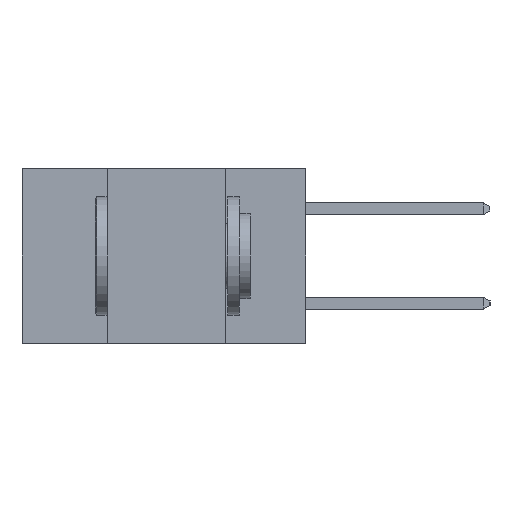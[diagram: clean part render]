
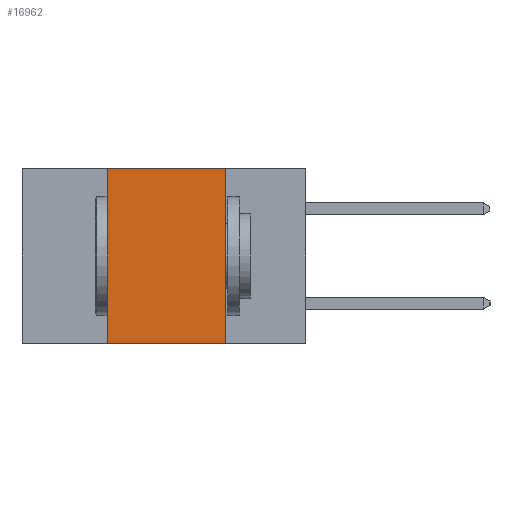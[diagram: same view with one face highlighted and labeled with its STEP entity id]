
A CAD part, left-side view. The second image highlights one B-rep face of the part: STEP entity #16962.
In plain terms, the highlighted planar face has unit normal (-1, 0, 0).
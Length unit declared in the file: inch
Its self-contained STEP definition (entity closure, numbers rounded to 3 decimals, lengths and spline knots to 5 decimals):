
#395 = CARTESIAN_POINT ( 'NONE',  ( 0., 0.17, -0.37 ) ) ;
#1537 = CARTESIAN_POINT ( 'NONE',  ( 0., 0.42, -0.37 ) ) ;
#2744 = VECTOR ( 'NONE', #6840, 39.37008 ) ;
#3295 = EDGE_CURVE ( 'NONE', #20723, #13925, #17741, .T. ) ;
#4956 = LINE ( 'NONE', #1537, #2744 ) ;
#6370 = ORIENTED_EDGE ( 'NONE', *, *, #20354, .F. ) ;
#6571 = VERTEX_POINT ( 'NONE', #9847 ) ;
#6707 = EDGE_CURVE ( 'NONE', #20723, #6571, #4956, .T. ) ;
#6840 = DIRECTION ( 'NONE',  ( 0., 0., 1. ) ) ;
#7305 = CARTESIAN_POINT ( 'NONE',  ( 0., 0.17, 0. ) ) ;
#7381 = DIRECTION ( 'NONE',  ( 0., 0., -1. ) ) ;
#7434 = ORIENTED_EDGE ( 'NONE', *, *, #18103, .F. ) ;
#7742 = LINE ( 'NONE', #17354, #16255 ) ;
#7825 = CARTESIAN_POINT ( 'NONE',  ( 0., 0.6, 0. ) ) ;
#8063 = FACE_OUTER_BOUND ( 'NONE', #19942, .T. ) ;
#9547 = DIRECTION ( 'NONE',  ( 1., 0., 0. ) ) ;
#9847 = CARTESIAN_POINT ( 'NONE',  ( 0., 0.42, 0. ) ) ;
#11132 = VERTEX_POINT ( 'NONE', #7305 ) ;
#11273 = CARTESIAN_POINT ( 'NONE',  ( 0., 0.6, -0.37 ) ) ;
#11319 = VECTOR ( 'NONE', #7381, 39.37008 ) ;
#11562 = DIRECTION ( 'NONE',  ( 0., -1., 0. ) ) ;
#12730 = VECTOR ( 'NONE', #11562, 39.37008 ) ;
#13925 = VERTEX_POINT ( 'NONE', #22145 ) ;
#15655 = DIRECTION ( 'NONE',  ( 0., -1., 0. ) ) ;
#16255 = VECTOR ( 'NONE', #15655, 39.37008 ) ;
#16962 = ADVANCED_FACE ( 'NONE', ( #8063 ), #17998, .F. ) ;
#17114 = AXIS2_PLACEMENT_3D ( 'NONE', #7825, #9547, #21385 ) ;
#17354 = CARTESIAN_POINT ( 'NONE',  ( 0., 0.6, 0. ) ) ;
#17741 = LINE ( 'NONE', #11273, #12730 ) ;
#17998 = PLANE ( 'NONE',  #17114 ) ;
#18085 = ORIENTED_EDGE ( 'NONE', *, *, #3295, .T. ) ;
#18103 = EDGE_CURVE ( 'NONE', #6571, #11132, #7742, .T. ) ;
#19942 = EDGE_LOOP ( 'NONE', ( #6370, #7434, #21500, #18085 ) ) ;
#20138 = CARTESIAN_POINT ( 'NONE',  ( 0., 0.42, -0.37 ) ) ;
#20300 = LINE ( 'NONE', #395, #11319 ) ;
#20354 = EDGE_CURVE ( 'NONE', #11132, #13925, #20300, .T. ) ;
#20723 = VERTEX_POINT ( 'NONE', #20138 ) ;
#21385 = DIRECTION ( 'NONE',  ( 0., 0., -1. ) ) ;
#21500 = ORIENTED_EDGE ( 'NONE', *, *, #6707, .F. ) ;
#22145 = CARTESIAN_POINT ( 'NONE',  ( 0., 0.17, -0.37 ) ) ;
